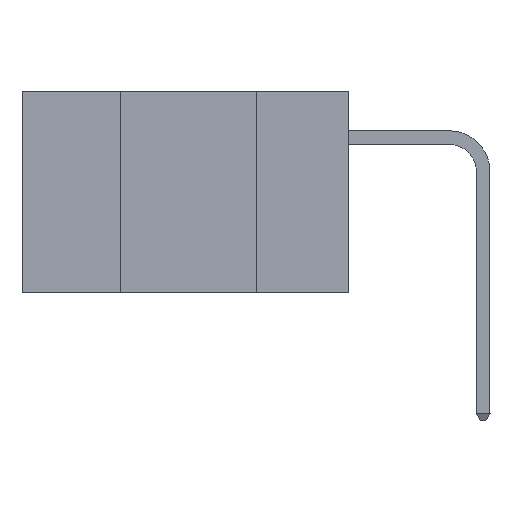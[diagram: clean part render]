
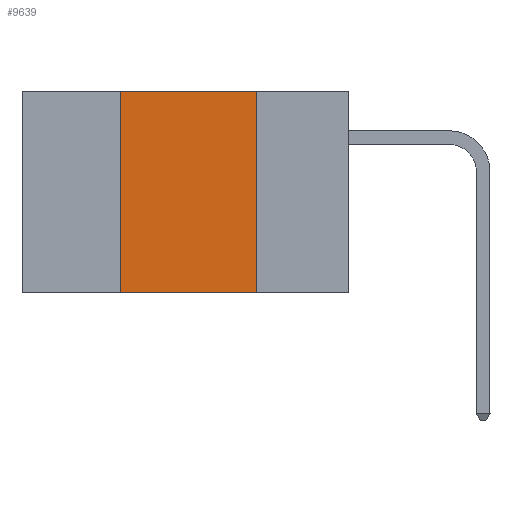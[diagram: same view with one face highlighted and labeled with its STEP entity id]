
A CAD part, left-side view. The second image highlights one B-rep face of the part: STEP entity #9639.
In plain terms, the highlighted planar face has unit normal (-1, 0, 0).
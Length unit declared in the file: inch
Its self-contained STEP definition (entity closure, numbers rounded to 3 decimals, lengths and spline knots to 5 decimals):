
#735 = LINE ( 'NONE', #15697, #9285 ) ;
#745 = CARTESIAN_POINT ( 'NONE',  ( 0., 0.17, -0.37 ) ) ;
#1257 = VERTEX_POINT ( 'NONE', #2033 ) ;
#1437 = VECTOR ( 'NONE', #10325, 39.37008 ) ;
#1829 = VERTEX_POINT ( 'NONE', #745 ) ;
#2033 = CARTESIAN_POINT ( 'NONE',  ( 0., 0.17, 0. ) ) ;
#2284 = DIRECTION ( 'NONE',  ( 0., 0., 1. ) ) ;
#4888 = DIRECTION ( 'NONE',  ( 0., 0., -1. ) ) ;
#5434 = DIRECTION ( 'NONE',  ( 0., 0., -1. ) ) ;
#6758 = ORIENTED_EDGE ( 'NONE', *, *, #15792, .T. ) ;
#8087 = LINE ( 'NONE', #13986, #23989 ) ;
#8116 = EDGE_CURVE ( 'NONE', #14135, #1257, #12197, .T. ) ;
#8805 = CARTESIAN_POINT ( 'NONE',  ( 0., 0.42, 0. ) ) ;
#9285 = VECTOR ( 'NONE', #15822, 39.37008 ) ;
#9499 = ORIENTED_EDGE ( 'NONE', *, *, #24698, .F. ) ;
#9565 = VECTOR ( 'NONE', #5434, 39.37008 ) ;
#9639 = ADVANCED_FACE ( 'NONE', ( #14068 ), #17967, .F. ) ;
#9662 = ORIENTED_EDGE ( 'NONE', *, *, #8116, .F. ) ;
#10325 = DIRECTION ( 'NONE',  ( 0., -1., 0. ) ) ;
#12197 = LINE ( 'NONE', #19858, #1437 ) ;
#12554 = EDGE_CURVE ( 'NONE', #1257, #1829, #13094, .T. ) ;
#12733 = AXIS2_PLACEMENT_3D ( 'NONE', #23733, #21980, #4888 ) ;
#13094 = LINE ( 'NONE', #16996, #9565 ) ;
#13986 = CARTESIAN_POINT ( 'NONE',  ( 0., 0.42, 0. ) ) ;
#14068 = FACE_OUTER_BOUND ( 'NONE', #15765, .T. ) ;
#14135 = VERTEX_POINT ( 'NONE', #8805 ) ;
#15697 = CARTESIAN_POINT ( 'NONE',  ( 0., 0.6, -0.37 ) ) ;
#15765 = EDGE_LOOP ( 'NONE', ( #20333, #9662, #9499, #6758 ) ) ;
#15792 = EDGE_CURVE ( 'NONE', #18301, #1829, #735, .T. ) ;
#15822 = DIRECTION ( 'NONE',  ( 0., -1., 0. ) ) ;
#16996 = CARTESIAN_POINT ( 'NONE',  ( 0., 0.17, 0. ) ) ;
#17967 = PLANE ( 'NONE',  #12733 ) ;
#18301 = VERTEX_POINT ( 'NONE', #24702 ) ;
#19858 = CARTESIAN_POINT ( 'NONE',  ( 0., 0.6, 0. ) ) ;
#20333 = ORIENTED_EDGE ( 'NONE', *, *, #12554, .F. ) ;
#21980 = DIRECTION ( 'NONE',  ( 1., 0., 0. ) ) ;
#23733 = CARTESIAN_POINT ( 'NONE',  ( 0., 0.6, 0. ) ) ;
#23989 = VECTOR ( 'NONE', #2284, 39.37008 ) ;
#24698 = EDGE_CURVE ( 'NONE', #18301, #14135, #8087, .T. ) ;
#24702 = CARTESIAN_POINT ( 'NONE',  ( 0., 0.42, -0.37 ) ) ;
